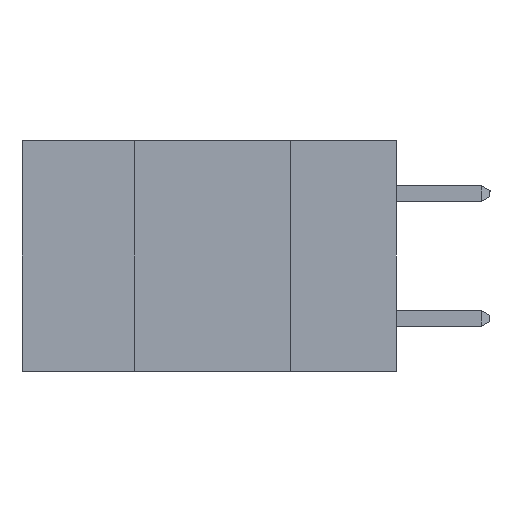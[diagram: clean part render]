
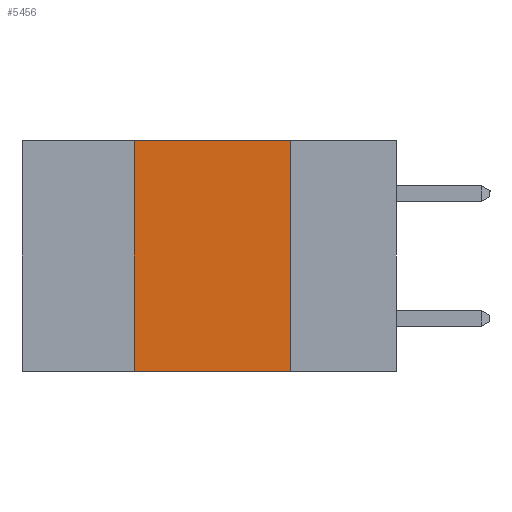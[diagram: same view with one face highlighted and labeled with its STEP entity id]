
A CAD part, left-side view. The second image highlights one B-rep face of the part: STEP entity #5456.
In plain terms, the highlighted planar face has unit normal (-1, 0, 0).
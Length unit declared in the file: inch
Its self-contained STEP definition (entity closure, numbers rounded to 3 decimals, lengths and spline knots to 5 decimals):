
#814 = CARTESIAN_POINT ( 'NONE',  ( 0., 0.17, -0.37 ) ) ;
#937 = DIRECTION ( 'NONE',  ( 0., 0., 1. ) ) ;
#1008 = VERTEX_POINT ( 'NONE', #814 ) ;
#1144 = ORIENTED_EDGE ( 'NONE', *, *, #9620, .T. ) ;
#2480 = EDGE_LOOP ( 'NONE', ( #5190, #11292, #8175, #1144 ) ) ;
#3472 = VECTOR ( 'NONE', #15470, 39.37008 ) ;
#3613 = LINE ( 'NONE', #16097, #11636 ) ;
#4772 = DIRECTION ( 'NONE',  ( 1., 0., 0. ) ) ;
#5161 = DIRECTION ( 'NONE',  ( 0., -1., 0. ) ) ;
#5190 = ORIENTED_EDGE ( 'NONE', *, *, #16429, .F. ) ;
#5268 = CARTESIAN_POINT ( 'NONE',  ( 0., 0.42, -0.37 ) ) ;
#5456 = ADVANCED_FACE ( 'NONE', ( #8276 ), #6889, .F. ) ;
#5864 = VERTEX_POINT ( 'NONE', #12276 ) ;
#5949 = DIRECTION ( 'NONE',  ( 0., 0., -1. ) ) ;
#6409 = VERTEX_POINT ( 'NONE', #15637 ) ;
#6889 = PLANE ( 'NONE',  #9578 ) ;
#7523 = VERTEX_POINT ( 'NONE', #9708 ) ;
#8175 = ORIENTED_EDGE ( 'NONE', *, *, #15267, .F. ) ;
#8276 = FACE_OUTER_BOUND ( 'NONE', #2480, .T. ) ;
#9160 = LINE ( 'NONE', #5268, #14577 ) ;
#9578 = AXIS2_PLACEMENT_3D ( 'NONE', #11370, #4772, #5949 ) ;
#9620 = EDGE_CURVE ( 'NONE', #7523, #1008, #17829, .T. ) ;
#9708 = CARTESIAN_POINT ( 'NONE',  ( 0., 0.42, -0.37 ) ) ;
#10124 = EDGE_CURVE ( 'NONE', #6409, #5864, #3613, .T. ) ;
#10168 = CARTESIAN_POINT ( 'NONE',  ( 0., 0.17, -0.37 ) ) ;
#10370 = CARTESIAN_POINT ( 'NONE',  ( 0., 0.6, -0.37 ) ) ;
#10552 = DIRECTION ( 'NONE',  ( 0., -1., 0. ) ) ;
#11292 = ORIENTED_EDGE ( 'NONE', *, *, #10124, .F. ) ;
#11370 = CARTESIAN_POINT ( 'NONE',  ( 0., 0.6, 0. ) ) ;
#11636 = VECTOR ( 'NONE', #5161, 39.37008 ) ;
#12276 = CARTESIAN_POINT ( 'NONE',  ( 0., 0.17, 0. ) ) ;
#14577 = VECTOR ( 'NONE', #937, 39.37008 ) ;
#15267 = EDGE_CURVE ( 'NONE', #7523, #6409, #9160, .T. ) ;
#15470 = DIRECTION ( 'NONE',  ( 0., 0., -1. ) ) ;
#15637 = CARTESIAN_POINT ( 'NONE',  ( 0., 0.42, 0. ) ) ;
#16097 = CARTESIAN_POINT ( 'NONE',  ( 0., 0.6, 0. ) ) ;
#16429 = EDGE_CURVE ( 'NONE', #5864, #1008, #17018, .T. ) ;
#16821 = VECTOR ( 'NONE', #10552, 39.37008 ) ;
#17018 = LINE ( 'NONE', #10168, #3472 ) ;
#17829 = LINE ( 'NONE', #10370, #16821 ) ;
